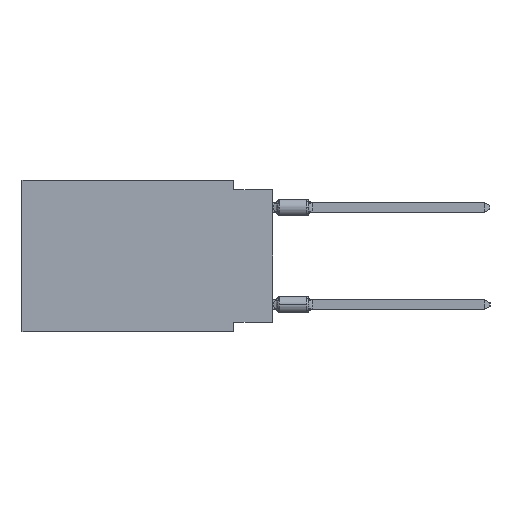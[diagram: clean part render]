
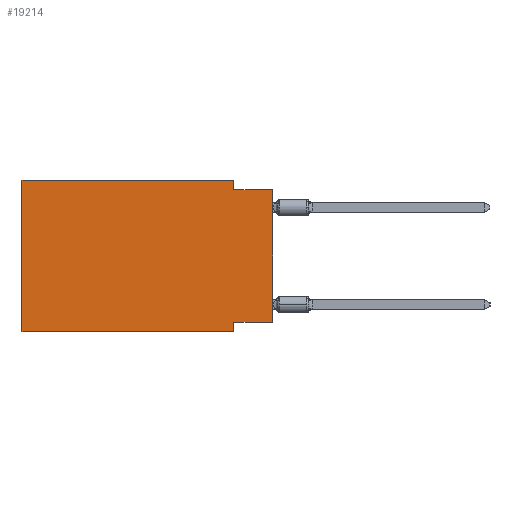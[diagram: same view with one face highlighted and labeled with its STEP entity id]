
A CAD part, left-side view. The second image highlights one B-rep face of the part: STEP entity #19214.
In plain terms, the highlighted planar face has unit normal (-1, 0, 0).
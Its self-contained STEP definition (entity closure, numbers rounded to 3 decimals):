
#121 = EDGE_CURVE ( 'NONE', #24064, #4419, #15049, .T. ) ;
#1312 = CARTESIAN_POINT ( 'NONE',  ( 0., 2.54, -0.635 ) ) ;
#2907 = CARTESIAN_POINT ( 'NONE',  ( 0., 2.54, -9.906 ) ) ;
#2933 = LINE ( 'NONE', #10710, #31346 ) ;
#3370 = LINE ( 'NONE', #12038, #35313 ) ;
#4419 = VERTEX_POINT ( 'NONE', #25681 ) ;
#5927 = VECTOR ( 'NONE', #22488, 1000. ) ;
#6227 = DIRECTION ( 'NONE',  ( 0., -1., 0. ) ) ;
#7220 = DIRECTION ( 'NONE',  ( 0., 0., 1. ) ) ;
#7426 = EDGE_CURVE ( 'NONE', #18590, #12933, #38501, .T. ) ;
#7956 = EDGE_CURVE ( 'NONE', #38999, #18590, #31252, .T. ) ;
#8156 = VERTEX_POINT ( 'NONE', #14042 ) ;
#9111 = VECTOR ( 'NONE', #40275, 1000. ) ;
#10064 = CARTESIAN_POINT ( 'NONE',  ( 0., 2.54, -9.271 ) ) ;
#10405 = ORIENTED_EDGE ( 'NONE', *, *, #26243, .T. ) ;
#10710 = CARTESIAN_POINT ( 'NONE',  ( 0., 0., -0.635 ) ) ;
#11664 = EDGE_CURVE ( 'NONE', #4419, #34896, #3370, .T. ) ;
#12038 = CARTESIAN_POINT ( 'NONE',  ( 0., 16.383, 0. ) ) ;
#12933 = VERTEX_POINT ( 'NONE', #25982 ) ;
#14042 = CARTESIAN_POINT ( 'NONE',  ( 0., 0., -0.635 ) ) ;
#14312 = AXIS2_PLACEMENT_3D ( 'NONE', #22241, #29779, #33543 ) ;
#15049 = LINE ( 'NONE', #40728, #9111 ) ;
#15516 = CARTESIAN_POINT ( 'NONE',  ( 0., 2.54, 0. ) ) ;
#17437 = VECTOR ( 'NONE', #6227, 1000. ) ;
#18590 = VERTEX_POINT ( 'NONE', #10064 ) ;
#18827 = ORIENTED_EDGE ( 'NONE', *, *, #7426, .F. ) ;
#18870 = VERTEX_POINT ( 'NONE', #1312 ) ;
#18994 = ORIENTED_EDGE ( 'NONE', *, *, #7956, .F. ) ;
#19214 = ADVANCED_FACE ( 'NONE', ( #26011 ), #44390, .F. ) ;
#22241 = CARTESIAN_POINT ( 'NONE',  ( 0., 16.383, 0. ) ) ;
#22488 = DIRECTION ( 'NONE',  ( 0., 0., -1. ) ) ;
#23186 = LINE ( 'NONE', #44894, #5927 ) ;
#23477 = DIRECTION ( 'NONE',  ( 0., 1., 0. ) ) ;
#23896 = CARTESIAN_POINT ( 'NONE',  ( 0., 16.383, -9.906 ) ) ;
#23943 = CARTESIAN_POINT ( 'NONE',  ( 0., 0., -9.271 ) ) ;
#24064 = VERTEX_POINT ( 'NONE', #32324 ) ;
#24349 = DIRECTION ( 'NONE',  ( 0., 0., -1. ) ) ;
#25681 = CARTESIAN_POINT ( 'NONE',  ( 0., 16.383, 0. ) ) ;
#25982 = CARTESIAN_POINT ( 'NONE',  ( 0., 2.54, -9.906 ) ) ;
#26011 = FACE_OUTER_BOUND ( 'NONE', #29235, .T. ) ;
#26243 = EDGE_CURVE ( 'NONE', #38999, #8156, #39522, .T. ) ;
#27667 = EDGE_CURVE ( 'NONE', #18870, #8156, #2933, .T. ) ;
#28862 = DIRECTION ( 'NONE',  ( 0., -1., 0. ) ) ;
#29235 = EDGE_LOOP ( 'NONE', ( #10405, #39443, #32207, #38201, #29882, #38585, #18827, #18994 ) ) ;
#29779 = DIRECTION ( 'NONE',  ( 1., 0., 0. ) ) ;
#29882 = ORIENTED_EDGE ( 'NONE', *, *, #121, .F. ) ;
#31207 = LINE ( 'NONE', #23896, #17437 ) ;
#31252 = LINE ( 'NONE', #23943, #45353 ) ;
#31346 = VECTOR ( 'NONE', #28862, 1000. ) ;
#32207 = ORIENTED_EDGE ( 'NONE', *, *, #36901, .F. ) ;
#32324 = CARTESIAN_POINT ( 'NONE',  ( 0., 16.383, -9.906 ) ) ;
#33543 = DIRECTION ( 'NONE',  ( 0., 0., -1. ) ) ;
#34896 = VERTEX_POINT ( 'NONE', #15516 ) ;
#35313 = VECTOR ( 'NONE', #39872, 1000. ) ;
#36901 = EDGE_CURVE ( 'NONE', #34896, #18870, #23186, .T. ) ;
#37913 = VECTOR ( 'NONE', #24349, 1000. ) ;
#38201 = ORIENTED_EDGE ( 'NONE', *, *, #11664, .F. ) ;
#38501 = LINE ( 'NONE', #2907, #37913 ) ;
#38585 = ORIENTED_EDGE ( 'NONE', *, *, #40504, .T. ) ;
#38999 = VERTEX_POINT ( 'NONE', #39510 ) ;
#39443 = ORIENTED_EDGE ( 'NONE', *, *, #27667, .F. ) ;
#39510 = CARTESIAN_POINT ( 'NONE',  ( 0., 0., -9.271 ) ) ;
#39522 = LINE ( 'NONE', #42359, #41890 ) ;
#39872 = DIRECTION ( 'NONE',  ( 0., -1., 0. ) ) ;
#40275 = DIRECTION ( 'NONE',  ( 0., 0., 1. ) ) ;
#40504 = EDGE_CURVE ( 'NONE', #24064, #12933, #31207, .T. ) ;
#40728 = CARTESIAN_POINT ( 'NONE',  ( 0., 16.383, 0. ) ) ;
#41890 = VECTOR ( 'NONE', #7220, 1000. ) ;
#42359 = CARTESIAN_POINT ( 'NONE',  ( 0., 0., 0. ) ) ;
#44390 = PLANE ( 'NONE',  #14312 ) ;
#44894 = CARTESIAN_POINT ( 'NONE',  ( 0., 2.54, 0. ) ) ;
#45353 = VECTOR ( 'NONE', #23477, 1000. ) ;
